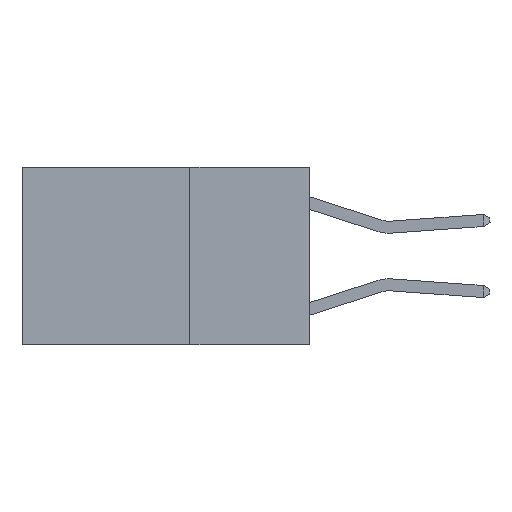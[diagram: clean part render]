
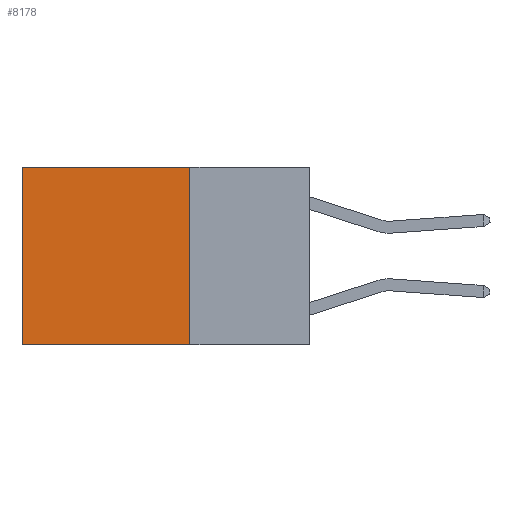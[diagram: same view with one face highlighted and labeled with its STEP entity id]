
A CAD part, left-side view. The second image highlights one B-rep face of the part: STEP entity #8178.
In plain terms, the highlighted planar face has unit normal (-1, 0, 0).
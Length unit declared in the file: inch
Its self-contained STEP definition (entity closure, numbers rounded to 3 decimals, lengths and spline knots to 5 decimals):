
#331 = VECTOR ( 'NONE', #3207, 39.37008 ) ;
#631 = LINE ( 'NONE', #9873, #7467 ) ;
#794 = VERTEX_POINT ( 'NONE', #3502 ) ;
#1106 = LINE ( 'NONE', #8735, #10080 ) ;
#1199 = LINE ( 'NONE', #10093, #331 ) ;
#1451 = VECTOR ( 'NONE', #1840, 39.37008 ) ;
#1812 = CARTESIAN_POINT ( 'NONE',  ( 0.2625, 0.25, 0. ) ) ;
#1840 = DIRECTION ( 'NONE',  ( 0., 1., 0. ) ) ;
#1862 = ORIENTED_EDGE ( 'NONE', *, *, #6561, .T. ) ;
#1996 = VERTEX_POINT ( 'NONE', #7158 ) ;
#2522 = VERTEX_POINT ( 'NONE', #3209 ) ;
#2964 = DIRECTION ( 'NONE',  ( 0., 0., -1. ) ) ;
#3207 = DIRECTION ( 'NONE',  ( 0., 1., 0. ) ) ;
#3209 = CARTESIAN_POINT ( 'NONE',  ( 0.2625, 0.6, 0. ) ) ;
#3502 = CARTESIAN_POINT ( 'NONE',  ( 0.2625, 0.25, -0.37 ) ) ;
#3844 = EDGE_CURVE ( 'NONE', #4859, #794, #631, .T. ) ;
#3976 = CARTESIAN_POINT ( 'NONE',  ( 0.2625, 0.25, 0. ) ) ;
#4804 = ORIENTED_EDGE ( 'NONE', *, *, #7741, .F. ) ;
#4834 = DIRECTION ( 'NONE',  ( 0., 0., -1. ) ) ;
#4859 = VERTEX_POINT ( 'NONE', #1812 ) ;
#4972 = AXIS2_PLACEMENT_3D ( 'NONE', #3976, #9965, #4834 ) ;
#5326 = EDGE_LOOP ( 'NONE', ( #1862, #4804, #10734, #10507 ) ) ;
#5433 = EDGE_CURVE ( 'NONE', #4859, #2522, #8506, .T. ) ;
#6185 = DIRECTION ( 'NONE',  ( 0., 0., -1. ) ) ;
#6561 = EDGE_CURVE ( 'NONE', #2522, #1996, #1106, .T. ) ;
#6592 = PLANE ( 'NONE',  #4972 ) ;
#7158 = CARTESIAN_POINT ( 'NONE',  ( 0.2625, 0.6, -0.37 ) ) ;
#7467 = VECTOR ( 'NONE', #2964, 39.37008 ) ;
#7741 = EDGE_CURVE ( 'NONE', #794, #1996, #1199, .T. ) ;
#8178 = ADVANCED_FACE ( 'NONE', ( #10617 ), #6592, .F. ) ;
#8506 = LINE ( 'NONE', #10444, #1451 ) ;
#8735 = CARTESIAN_POINT ( 'NONE',  ( 0.2625, 0.6, 0. ) ) ;
#9873 = CARTESIAN_POINT ( 'NONE',  ( 0.2625, 0.25, 0. ) ) ;
#9965 = DIRECTION ( 'NONE',  ( 1., 0., 0. ) ) ;
#10080 = VECTOR ( 'NONE', #6185, 39.37008 ) ;
#10093 = CARTESIAN_POINT ( 'NONE',  ( 0.2625, 0.25, -0.37 ) ) ;
#10444 = CARTESIAN_POINT ( 'NONE',  ( 0.2625, 0.25, 0. ) ) ;
#10507 = ORIENTED_EDGE ( 'NONE', *, *, #5433, .T. ) ;
#10617 = FACE_OUTER_BOUND ( 'NONE', #5326, .T. ) ;
#10734 = ORIENTED_EDGE ( 'NONE', *, *, #3844, .F. ) ;
